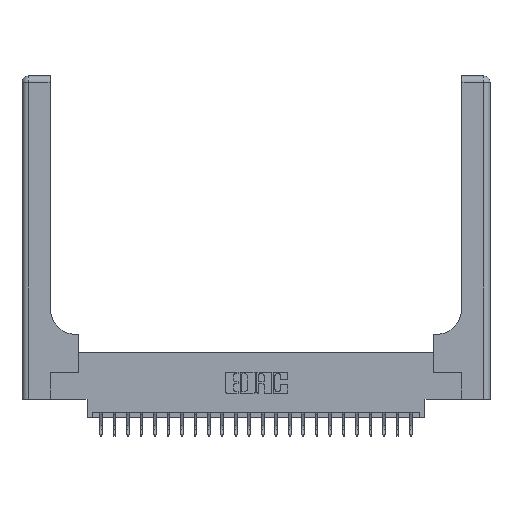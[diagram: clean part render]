
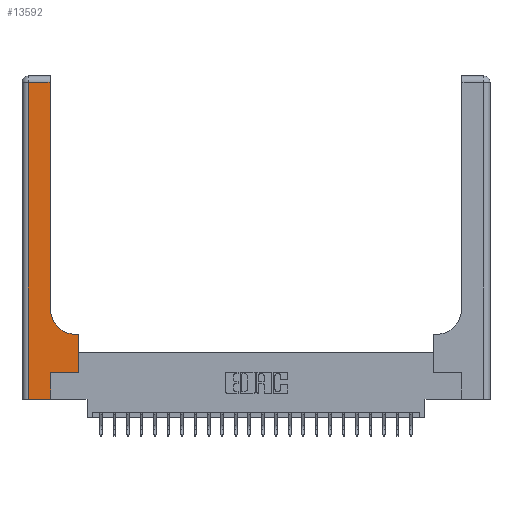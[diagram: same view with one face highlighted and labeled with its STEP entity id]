
A CAD part, top view. The second image highlights one B-rep face of the part: STEP entity #13592.
In plain terms, the highlighted planar face has unit normal (0, 0, 1).
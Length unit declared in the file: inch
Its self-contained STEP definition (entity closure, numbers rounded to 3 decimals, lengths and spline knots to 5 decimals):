
#226 = CARTESIAN_POINT ( 'NONE',  ( 0.26, 0.85, 0.37 ) ) ;
#780 = CARTESIAN_POINT ( 'NONE',  ( 0.528, 0.6, 0.37 ) ) ;
#781 = VERTEX_POINT ( 'NONE', #16724 ) ;
#1262 = CARTESIAN_POINT ( 'NONE',  ( 0.06, 3., 0.37 ) ) ;
#1361 = LINE ( 'NONE', #20697, #20805 ) ;
#1616 = ORIENTED_EDGE ( 'NONE', *, *, #21656, .T. ) ;
#1746 = LINE ( 'NONE', #16458, #6088 ) ;
#2027 = CARTESIAN_POINT ( 'NONE',  ( 0.51, 0.6, 0.37 ) ) ;
#2428 = DIRECTION ( 'NONE',  ( -1., 0., 0. ) ) ;
#2490 = ORIENTED_EDGE ( 'NONE', *, *, #13334, .T. ) ;
#3132 = DIRECTION ( 'NONE',  ( 0., -1., 0. ) ) ;
#3170 = CARTESIAN_POINT ( 'NONE',  ( 0.265, 0., 0.37 ) ) ;
#3507 = VECTOR ( 'NONE', #10046, 39.37008 ) ;
#3529 = CARTESIAN_POINT ( 'NONE',  ( 0.265, 0.25, 0.37 ) ) ;
#3662 = ORIENTED_EDGE ( 'NONE', *, *, #4284, .T. ) ;
#3759 = EDGE_CURVE ( 'NONE', #17364, #9241, #8403, .T. ) ;
#4113 = DIRECTION ( 'NONE',  ( 0., 0., -1. ) ) ;
#4284 = EDGE_CURVE ( 'NONE', #11226, #15597, #16391, .T. ) ;
#4293 = VECTOR ( 'NONE', #3132, 39.37008 ) ;
#4351 = CARTESIAN_POINT ( 'NONE',  ( 0.26, 3., 0.37 ) ) ;
#5337 = EDGE_CURVE ( 'NONE', #9241, #7101, #17950, .T. ) ;
#5785 = CARTESIAN_POINT ( 'NONE',  ( 0., 3., 0.37 ) ) ;
#6088 = VECTOR ( 'NONE', #7331, 39.37008 ) ;
#7101 = VERTEX_POINT ( 'NONE', #10291 ) ;
#7331 = DIRECTION ( 'NONE',  ( -1., 0., 0. ) ) ;
#7623 = DIRECTION ( 'NONE',  ( 0., 0., -1. ) ) ;
#7732 = VECTOR ( 'NONE', #20778, 39.37008 ) ;
#7987 = ORIENTED_EDGE ( 'NONE', *, *, #11403, .T. ) ;
#8359 = DIRECTION ( 'NONE',  ( 0., 1., 0. ) ) ;
#8402 = VECTOR ( 'NONE', #8359, 39.37008 ) ;
#8403 = LINE ( 'NONE', #20868, #3507 ) ;
#8941 = VERTEX_POINT ( 'NONE', #10605 ) ;
#9241 = VERTEX_POINT ( 'NONE', #9625 ) ;
#9625 = CARTESIAN_POINT ( 'NONE',  ( 0.265, 0., 0.37 ) ) ;
#9715 = EDGE_CURVE ( 'NONE', #8941, #21171, #1746, .T. ) ;
#10046 = DIRECTION ( 'NONE',  ( 1., 0., 0. ) ) ;
#10201 = EDGE_LOOP ( 'NONE', ( #1616, #22155, #13133, #23268, #14846, #16568, #2490, #7987, #3662 ) ) ;
#10291 = CARTESIAN_POINT ( 'NONE',  ( 0.265, 0.25, 0.37 ) ) ;
#10605 = CARTESIAN_POINT ( 'NONE',  ( 0.26, 2.94, 0.37 ) ) ;
#11226 = VERTEX_POINT ( 'NONE', #2027 ) ;
#11330 = LINE ( 'NONE', #3529, #19823 ) ;
#11403 = EDGE_CURVE ( 'NONE', #23616, #11226, #1361, .T. ) ;
#12045 = CARTESIAN_POINT ( 'NONE',  ( 0.528, 0.25, 0.37 ) ) ;
#12279 = EDGE_CURVE ( 'NONE', #7101, #781, #11330, .T. ) ;
#12525 = CARTESIAN_POINT ( 'NONE',  ( 0.06, 0., 0.37 ) ) ;
#12599 = LINE ( 'NONE', #4351, #7732 ) ;
#12854 = CARTESIAN_POINT ( 'NONE',  ( 0.06, 2.94, 0.37 ) ) ;
#13133 = ORIENTED_EDGE ( 'NONE', *, *, #14594, .T. ) ;
#13334 = EDGE_CURVE ( 'NONE', #781, #23616, #18644, .T. ) ;
#13592 = ADVANCED_FACE ( 'NONE', ( #23113 ), #16726, .F. ) ;
#14174 = DIRECTION ( 'NONE',  ( 0., 1., 0. ) ) ;
#14516 = DIRECTION ( 'NONE',  ( 1., 0., 0. ) ) ;
#14594 = EDGE_CURVE ( 'NONE', #21171, #17364, #17740, .T. ) ;
#14846 = ORIENTED_EDGE ( 'NONE', *, *, #5337, .T. ) ;
#15093 = CARTESIAN_POINT ( 'NONE',  ( 0.51, 0.85, 0.37 ) ) ;
#15597 = VERTEX_POINT ( 'NONE', #226 ) ;
#15819 = AXIS2_PLACEMENT_3D ( 'NONE', #15093, #4113, #16921 ) ;
#16391 = CIRCLE ( 'NONE', #15819, 0.25 ) ;
#16458 = CARTESIAN_POINT ( 'NONE',  ( 0., 2.94, 0.37 ) ) ;
#16568 = ORIENTED_EDGE ( 'NONE', *, *, #12279, .T. ) ;
#16724 = CARTESIAN_POINT ( 'NONE',  ( 0.528, 0.25, 0.37 ) ) ;
#16726 = PLANE ( 'NONE',  #18504 ) ;
#16921 = DIRECTION ( 'NONE',  ( 1., 0., 0. ) ) ;
#17364 = VERTEX_POINT ( 'NONE', #12525 ) ;
#17740 = LINE ( 'NONE', #1262, #4293 ) ;
#17950 = LINE ( 'NONE', #3170, #21609 ) ;
#18504 = AXIS2_PLACEMENT_3D ( 'NONE', #5785, #7623, #20328 ) ;
#18644 = LINE ( 'NONE', #12045, #8402 ) ;
#19823 = VECTOR ( 'NONE', #14516, 39.37008 ) ;
#20328 = DIRECTION ( 'NONE',  ( -1., 0., 0. ) ) ;
#20697 = CARTESIAN_POINT ( 'NONE',  ( 0.26, 0.6, 0.37 ) ) ;
#20778 = DIRECTION ( 'NONE',  ( 0., 1., 0. ) ) ;
#20805 = VECTOR ( 'NONE', #2428, 39.37008 ) ;
#20868 = CARTESIAN_POINT ( 'NONE',  ( 0., 0., 0.37 ) ) ;
#21171 = VERTEX_POINT ( 'NONE', #12854 ) ;
#21609 = VECTOR ( 'NONE', #14174, 39.37008 ) ;
#21656 = EDGE_CURVE ( 'NONE', #15597, #8941, #12599, .T. ) ;
#22155 = ORIENTED_EDGE ( 'NONE', *, *, #9715, .T. ) ;
#23113 = FACE_OUTER_BOUND ( 'NONE', #10201, .T. ) ;
#23268 = ORIENTED_EDGE ( 'NONE', *, *, #3759, .T. ) ;
#23616 = VERTEX_POINT ( 'NONE', #780 ) ;
